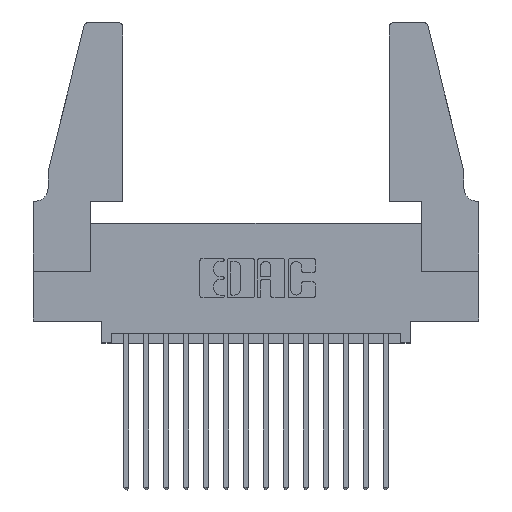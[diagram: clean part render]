
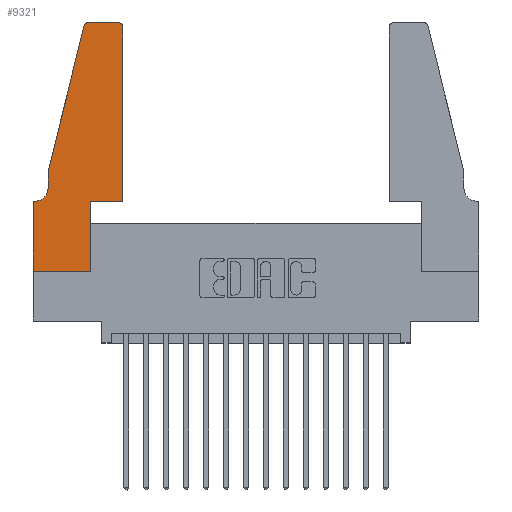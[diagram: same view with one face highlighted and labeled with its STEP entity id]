
A CAD part, top view. The second image highlights one B-rep face of the part: STEP entity #9321.
In plain terms, the highlighted planar face has unit normal (0, 0, 1).
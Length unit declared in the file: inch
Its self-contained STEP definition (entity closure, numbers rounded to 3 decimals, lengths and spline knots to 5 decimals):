
#360 = VERTEX_POINT ( 'NONE', #6357 ) ;
#398 = EDGE_CURVE ( 'NONE', #3503, #6623, #15175, .T. ) ;
#1611 = DIRECTION ( 'NONE',  ( 0., 1., 0. ) ) ;
#1715 = EDGE_CURVE ( 'NONE', #8006, #13646, #11707, .T. ) ;
#2045 = CARTESIAN_POINT ( 'NONE',  ( 0.2865, 0.35, 0.37 ) ) ;
#2089 = CARTESIAN_POINT ( 'NONE',  ( 0.0055, 0.42, 0.37 ) ) ;
#2420 = DIRECTION ( 'NONE',  ( 0., -1., 0. ) ) ;
#2458 = EDGE_CURVE ( 'NONE', #3680, #7310, #14186, .T. ) ;
#2524 = CARTESIAN_POINT ( 'NONE',  ( 0.0755, 0.5, 0.37 ) ) ;
#2924 = VERTEX_POINT ( 'NONE', #16135 ) ;
#3115 = VECTOR ( 'NONE', #1611, 39.37008 ) ;
#3170 = CARTESIAN_POINT ( 'NONE',  ( 0., 0.35, 0.37 ) ) ;
#3360 = CIRCLE ( 'NONE', #16212, 0.03 ) ;
#3503 = VERTEX_POINT ( 'NONE', #11687 ) ;
#3669 = EDGE_CURVE ( 'NONE', #6623, #4696, #9569, .T. ) ;
#3680 = VERTEX_POINT ( 'NONE', #14391 ) ;
#3878 = LINE ( 'NONE', #15027, #6164 ) ;
#3967 = VECTOR ( 'NONE', #6569, 39.37008 ) ;
#4395 = CIRCLE ( 'NONE', #16965, 0.03 ) ;
#4614 = CARTESIAN_POINT ( 'NONE',  ( 0.0755, 0.35, 0.37 ) ) ;
#4696 = VERTEX_POINT ( 'NONE', #2045 ) ;
#4834 = DIRECTION ( 'NONE',  ( -1., 0., 0. ) ) ;
#4842 = ORIENTED_EDGE ( 'NONE', *, *, #8105, .T. ) ;
#5022 = CARTESIAN_POINT ( 'NONE',  ( 0., 0., 0.37 ) ) ;
#5094 = DIRECTION ( 'NONE',  ( -0.239, -0.971, 0. ) ) ;
#5277 = DIRECTION ( 'NONE',  ( 1., 0., 0. ) ) ;
#5579 = ORIENTED_EDGE ( 'NONE', *, *, #1715, .T. ) ;
#5665 = CARTESIAN_POINT ( 'NONE',  ( 0.4205, 1.25, 0.37 ) ) ;
#5690 = CARTESIAN_POINT ( 'NONE',  ( 0.4505, 0.35, 0.37 ) ) ;
#5709 = VECTOR ( 'NONE', #2420, 39.37008 ) ;
#5874 = ORIENTED_EDGE ( 'NONE', *, *, #10854, .T. ) ;
#6068 = VECTOR ( 'NONE', #9335, 39.37008 ) ;
#6148 = EDGE_CURVE ( 'NONE', #13646, #3680, #7282, .T. ) ;
#6164 = VECTOR ( 'NONE', #12392, 39.37008 ) ;
#6357 = CARTESIAN_POINT ( 'NONE',  ( 0.284, 1.25, 0.37 ) ) ;
#6569 = DIRECTION ( 'NONE',  ( 1., 0., 0. ) ) ;
#6623 = VERTEX_POINT ( 'NONE', #10491 ) ;
#6773 = DIRECTION ( 'NONE',  ( 0., 0., 1. ) ) ;
#7071 = CARTESIAN_POINT ( 'NONE',  ( 0., 0., 0.37 ) ) ;
#7121 = DIRECTION ( 'NONE',  ( -1., 0., 0. ) ) ;
#7282 = LINE ( 'NONE', #12514, #9502 ) ;
#7310 = VERTEX_POINT ( 'NONE', #8963 ) ;
#8006 = VERTEX_POINT ( 'NONE', #15396 ) ;
#8034 = ORIENTED_EDGE ( 'NONE', *, *, #3669, .T. ) ;
#8105 = EDGE_CURVE ( 'NONE', #10569, #3503, #9826, .T. ) ;
#8113 = ORIENTED_EDGE ( 'NONE', *, *, #398, .T. ) ;
#8199 = DIRECTION ( 'NONE',  ( 1., 0., 0. ) ) ;
#8598 = ORIENTED_EDGE ( 'NONE', *, *, #13342, .T. ) ;
#8963 = CARTESIAN_POINT ( 'NONE',  ( 0.0055, 0.35, 0.37 ) ) ;
#9321 = ADVANCED_FACE ( 'NONE', ( #10594 ), #9446, .T. ) ;
#9335 = DIRECTION ( 'NONE',  ( 1., 0., 0. ) ) ;
#9432 = VERTEX_POINT ( 'NONE', #5665 ) ;
#9446 = PLANE ( 'NONE',  #10411 ) ;
#9502 = VECTOR ( 'NONE', #12566, 39.37008 ) ;
#9569 = LINE ( 'NONE', #14273, #12263 ) ;
#9826 = LINE ( 'NONE', #5022, #5709 ) ;
#9918 = CARTESIAN_POINT ( 'NONE',  ( 0.4505, 0.35, 0.37 ) ) ;
#9994 = EDGE_CURVE ( 'NONE', #2924, #9432, #3360, .T. ) ;
#10411 = AXIS2_PLACEMENT_3D ( 'NONE', #10785, #6773, #8199 ) ;
#10489 = ORIENTED_EDGE ( 'NONE', *, *, #15304, .T. ) ;
#10491 = CARTESIAN_POINT ( 'NONE',  ( 0.2865, 0., 0.37 ) ) ;
#10523 = CARTESIAN_POINT ( 'NONE',  ( 0.4205, 1.22, 0.37 ) ) ;
#10569 = VERTEX_POINT ( 'NONE', #3170 ) ;
#10570 = EDGE_CURVE ( 'NONE', #7310, #10569, #16764, .T. ) ;
#10594 = FACE_OUTER_BOUND ( 'NONE', #12154, .T. ) ;
#10754 = EDGE_CURVE ( 'NONE', #360, #8006, #4395, .T. ) ;
#10769 = VECTOR ( 'NONE', #7121, 39.37008 ) ;
#10785 = CARTESIAN_POINT ( 'NONE',  ( 0., 0.35, 0.37 ) ) ;
#10854 = EDGE_CURVE ( 'NONE', #4696, #14646, #16746, .T. ) ;
#10941 = CARTESIAN_POINT ( 'NONE',  ( 0.284, 1.22, 0.37 ) ) ;
#11074 = ORIENTED_EDGE ( 'NONE', *, *, #9994, .T. ) ;
#11078 = ORIENTED_EDGE ( 'NONE', *, *, #10570, .T. ) ;
#11508 = CARTESIAN_POINT ( 'NONE',  ( 0.0755, 0.5, 0.37 ) ) ;
#11536 = DIRECTION ( 'NONE',  ( 0., 1., 0. ) ) ;
#11687 = CARTESIAN_POINT ( 'NONE',  ( 0., 0., 0.37 ) ) ;
#11707 = LINE ( 'NONE', #11508, #12118 ) ;
#12118 = VECTOR ( 'NONE', #5094, 39.37008 ) ;
#12154 = EDGE_LOOP ( 'NONE', ( #8598, #16255, #5579, #14227, #16601, #11078, #4842, #8113, #8034, #5874, #10489, #11074 ) ) ;
#12263 = VECTOR ( 'NONE', #11536, 39.37008 ) ;
#12392 = DIRECTION ( 'NONE',  ( -1., 0., 0. ) ) ;
#12514 = CARTESIAN_POINT ( 'NONE',  ( 0.0755, 0.5, 0.37 ) ) ;
#12566 = DIRECTION ( 'NONE',  ( 0., -1., 0. ) ) ;
#13182 = DIRECTION ( 'NONE',  ( 1., 0., 0. ) ) ;
#13342 = EDGE_CURVE ( 'NONE', #9432, #360, #3878, .T. ) ;
#13404 = CARTESIAN_POINT ( 'NONE',  ( 0.4505, 0.35, 0.37 ) ) ;
#13646 = VERTEX_POINT ( 'NONE', #2524 ) ;
#13659 = LINE ( 'NONE', #13404, #3115 ) ;
#13666 = DIRECTION ( 'NONE',  ( 0., 0., 1. ) ) ;
#14186 = CIRCLE ( 'NONE', #15560, 0.07 ) ;
#14227 = ORIENTED_EDGE ( 'NONE', *, *, #6148, .T. ) ;
#14273 = CARTESIAN_POINT ( 'NONE',  ( 0.2865, 0.35, 0.37 ) ) ;
#14381 = DIRECTION ( 'NONE',  ( 0., 0., 1. ) ) ;
#14391 = CARTESIAN_POINT ( 'NONE',  ( 0.0755, 0.42, 0.37 ) ) ;
#14646 = VERTEX_POINT ( 'NONE', #9918 ) ;
#15027 = CARTESIAN_POINT ( 'NONE',  ( 0.2605, 1.25, 0.37 ) ) ;
#15175 = LINE ( 'NONE', #7071, #6068 ) ;
#15304 = EDGE_CURVE ( 'NONE', #14646, #2924, #13659, .T. ) ;
#15396 = CARTESIAN_POINT ( 'NONE',  ( 0.25487, 1.22718, 0.37 ) ) ;
#15560 = AXIS2_PLACEMENT_3D ( 'NONE', #2089, #16654, #4834 ) ;
#16135 = CARTESIAN_POINT ( 'NONE',  ( 0.4505, 1.22, 0.37 ) ) ;
#16212 = AXIS2_PLACEMENT_3D ( 'NONE', #10523, #14381, #13182 ) ;
#16255 = ORIENTED_EDGE ( 'NONE', *, *, #10754, .T. ) ;
#16601 = ORIENTED_EDGE ( 'NONE', *, *, #2458, .T. ) ;
#16654 = DIRECTION ( 'NONE',  ( 0., 0., -1. ) ) ;
#16746 = LINE ( 'NONE', #5690, #3967 ) ;
#16764 = LINE ( 'NONE', #4614, #10769 ) ;
#16965 = AXIS2_PLACEMENT_3D ( 'NONE', #10941, #13666, #5277 ) ;
